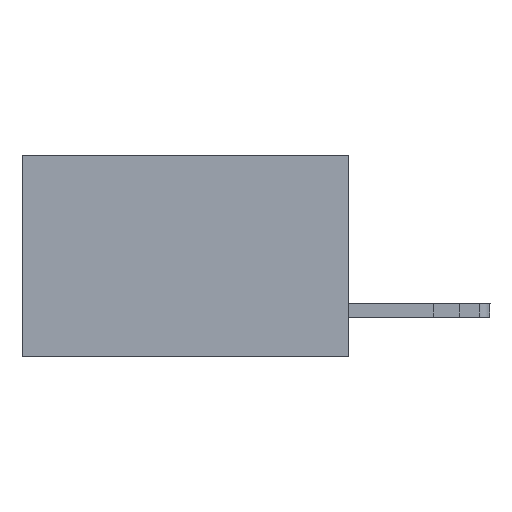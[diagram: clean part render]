
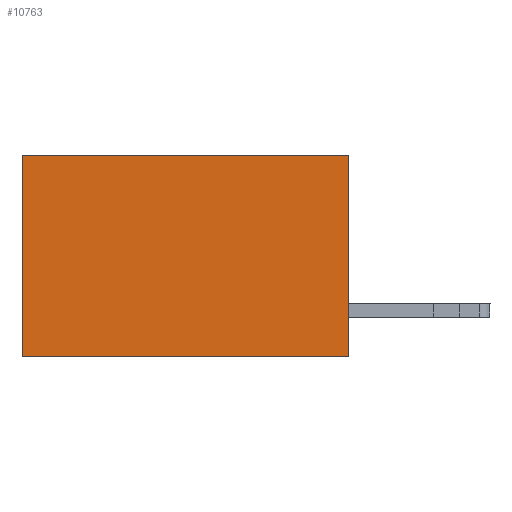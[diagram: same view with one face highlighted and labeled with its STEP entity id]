
A CAD part, left-side view. The second image highlights one B-rep face of the part: STEP entity #10763.
In plain terms, the highlighted planar face has unit normal (-1, 0, 0).
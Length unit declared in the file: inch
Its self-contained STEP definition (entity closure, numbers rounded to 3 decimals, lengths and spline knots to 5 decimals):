
#50 = ORIENTED_EDGE ( 'NONE', *, *, #12263, .T. ) ;
#418 = CARTESIAN_POINT ( 'NONE',  ( 0.2615, 0.6, -0.37 ) ) ;
#501 = DIRECTION ( 'NONE',  ( 1., 0., 0. ) ) ;
#548 = CARTESIAN_POINT ( 'NONE',  ( 0.2615, 0., -0.37 ) ) ;
#722 = VERTEX_POINT ( 'NONE', #418 ) ;
#765 = EDGE_CURVE ( 'NONE', #9993, #4568, #9099, .T. ) ;
#1400 = FACE_OUTER_BOUND ( 'NONE', #3087, .T. ) ;
#1970 = CARTESIAN_POINT ( 'NONE',  ( 0.2615, 0.6, 0. ) ) ;
#2137 = VECTOR ( 'NONE', #12169, 39.37008 ) ;
#2495 = DIRECTION ( 'NONE',  ( 0., 0., -1. ) ) ;
#3087 = EDGE_LOOP ( 'NONE', ( #50, #3713, #11733, #9256 ) ) ;
#3460 = DIRECTION ( 'NONE',  ( 0., 0., -1. ) ) ;
#3694 = DIRECTION ( 'NONE',  ( 0., 1., 0. ) ) ;
#3713 = ORIENTED_EDGE ( 'NONE', *, *, #3902, .F. ) ;
#3902 = EDGE_CURVE ( 'NONE', #4568, #722, #9189, .T. ) ;
#4450 = LINE ( 'NONE', #8364, #2137 ) ;
#4568 = VERTEX_POINT ( 'NONE', #4732 ) ;
#4732 = CARTESIAN_POINT ( 'NONE',  ( 0.2615, 0., -0.37 ) ) ;
#4765 = VECTOR ( 'NONE', #2495, 39.37008 ) ;
#5192 = CARTESIAN_POINT ( 'NONE',  ( 0.2615, 0., -0.37 ) ) ;
#6620 = VERTEX_POINT ( 'NONE', #1970 ) ;
#6895 = VECTOR ( 'NONE', #7832, 39.37008 ) ;
#7084 = AXIS2_PLACEMENT_3D ( 'NONE', #5192, #501, #3460 ) ;
#7528 = CARTESIAN_POINT ( 'NONE',  ( 0.2615, 0., 0. ) ) ;
#7832 = DIRECTION ( 'NONE',  ( 0., 1., 0. ) ) ;
#8364 = CARTESIAN_POINT ( 'NONE',  ( 0.2615, 0.6, -0.37 ) ) ;
#8494 = VECTOR ( 'NONE', #3694, 39.37008 ) ;
#8716 = CARTESIAN_POINT ( 'NONE',  ( 0.2615, 0., 0. ) ) ;
#9099 = LINE ( 'NONE', #548, #4765 ) ;
#9189 = LINE ( 'NONE', #9366, #8494 ) ;
#9256 = ORIENTED_EDGE ( 'NONE', *, *, #11685, .T. ) ;
#9366 = CARTESIAN_POINT ( 'NONE',  ( 0.2615, 0., -0.37 ) ) ;
#9993 = VERTEX_POINT ( 'NONE', #7528 ) ;
#10763 = ADVANCED_FACE ( 'NONE', ( #1400 ), #11924, .F. ) ;
#10841 = LINE ( 'NONE', #8716, #6895 ) ;
#11685 = EDGE_CURVE ( 'NONE', #9993, #6620, #10841, .T. ) ;
#11733 = ORIENTED_EDGE ( 'NONE', *, *, #765, .F. ) ;
#11924 = PLANE ( 'NONE',  #7084 ) ;
#12169 = DIRECTION ( 'NONE',  ( 0., 0., -1. ) ) ;
#12263 = EDGE_CURVE ( 'NONE', #6620, #722, #4450, .T. ) ;
